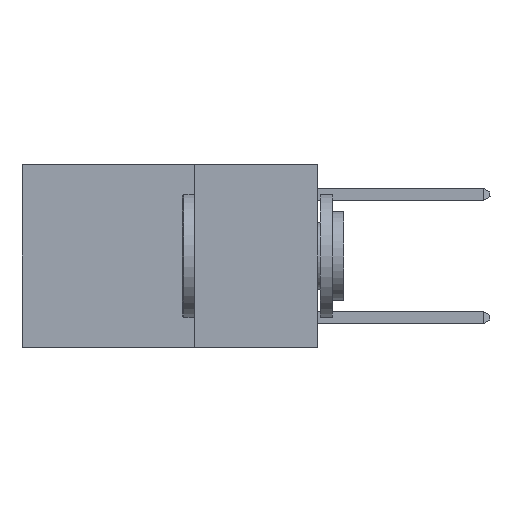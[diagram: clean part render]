
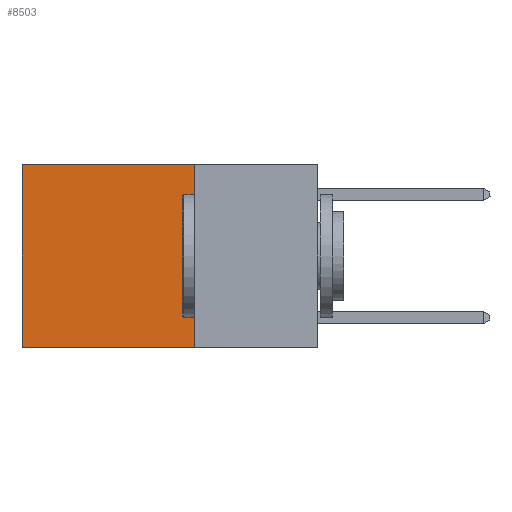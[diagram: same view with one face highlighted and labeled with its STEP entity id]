
A CAD part, left-side view. The second image highlights one B-rep face of the part: STEP entity #8503.
In plain terms, the highlighted planar face has unit normal (-1, 0, 0).
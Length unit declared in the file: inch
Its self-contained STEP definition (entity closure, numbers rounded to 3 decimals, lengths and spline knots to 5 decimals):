
#162 = EDGE_CURVE ( 'NONE', #11792, #12415, #6835, .T. ) ;
#173 = VERTEX_POINT ( 'NONE', #13407 ) ;
#337 = VECTOR ( 'NONE', #4622, 39.37008 ) ;
#754 = VECTOR ( 'NONE', #9155, 39.37008 ) ;
#1917 = CARTESIAN_POINT ( 'NONE',  ( 0.2625, 0.6, 0. ) ) ;
#2096 = LINE ( 'NONE', #6456, #10436 ) ;
#2974 = CARTESIAN_POINT ( 'NONE',  ( 0.2625, 0.25, -0.37 ) ) ;
#4622 = DIRECTION ( 'NONE',  ( 0., 0., -1. ) ) ;
#4987 = EDGE_LOOP ( 'NONE', ( #7368, #11916, #6383, #11552 ) ) ;
#5066 = LINE ( 'NONE', #2974, #9304 ) ;
#6060 = CARTESIAN_POINT ( 'NONE',  ( 0.2625, 0.25, -0.37 ) ) ;
#6383 = ORIENTED_EDGE ( 'NONE', *, *, #162, .F. ) ;
#6408 = AXIS2_PLACEMENT_3D ( 'NONE', #12362, #9420, #11352 ) ;
#6456 = CARTESIAN_POINT ( 'NONE',  ( 0.2625, 0.25, 0. ) ) ;
#6835 = LINE ( 'NONE', #9084, #754 ) ;
#6891 = EDGE_CURVE ( 'NONE', #11792, #173, #2096, .T. ) ;
#7116 = FACE_OUTER_BOUND ( 'NONE', #4987, .T. ) ;
#7368 = ORIENTED_EDGE ( 'NONE', *, *, #12597, .T. ) ;
#7609 = EDGE_CURVE ( 'NONE', #12415, #7633, #5066, .T. ) ;
#7633 = VERTEX_POINT ( 'NONE', #11600 ) ;
#8503 = ADVANCED_FACE ( 'NONE', ( #7116 ), #11562, .F. ) ;
#9084 = CARTESIAN_POINT ( 'NONE',  ( 0.2625, 0.25, 0. ) ) ;
#9155 = DIRECTION ( 'NONE',  ( 0., 0., -1. ) ) ;
#9304 = VECTOR ( 'NONE', #9383, 39.37008 ) ;
#9383 = DIRECTION ( 'NONE',  ( 0., 1., 0. ) ) ;
#9420 = DIRECTION ( 'NONE',  ( 1., 0., 0. ) ) ;
#9696 = DIRECTION ( 'NONE',  ( 0., 1., 0. ) ) ;
#10436 = VECTOR ( 'NONE', #9696, 39.37008 ) ;
#11352 = DIRECTION ( 'NONE',  ( 0., 0., -1. ) ) ;
#11552 = ORIENTED_EDGE ( 'NONE', *, *, #6891, .T. ) ;
#11562 = PLANE ( 'NONE',  #6408 ) ;
#11600 = CARTESIAN_POINT ( 'NONE',  ( 0.2625, 0.6, -0.37 ) ) ;
#11661 = LINE ( 'NONE', #1917, #337 ) ;
#11792 = VERTEX_POINT ( 'NONE', #12217 ) ;
#11916 = ORIENTED_EDGE ( 'NONE', *, *, #7609, .F. ) ;
#12217 = CARTESIAN_POINT ( 'NONE',  ( 0.2625, 0.25, 0. ) ) ;
#12362 = CARTESIAN_POINT ( 'NONE',  ( 0.2625, 0.25, 0. ) ) ;
#12415 = VERTEX_POINT ( 'NONE', #6060 ) ;
#12597 = EDGE_CURVE ( 'NONE', #173, #7633, #11661, .T. ) ;
#13407 = CARTESIAN_POINT ( 'NONE',  ( 0.2625, 0.6, 0. ) ) ;
